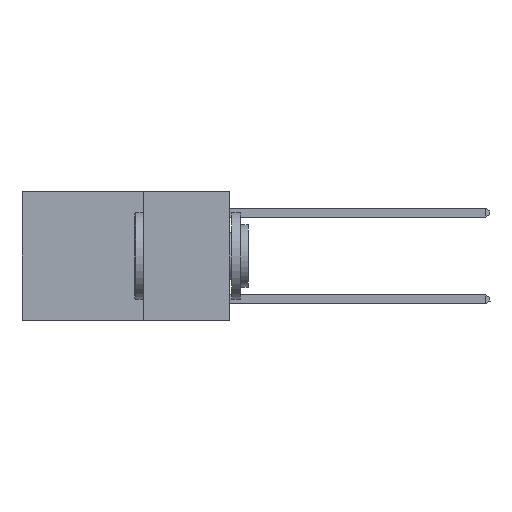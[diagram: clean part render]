
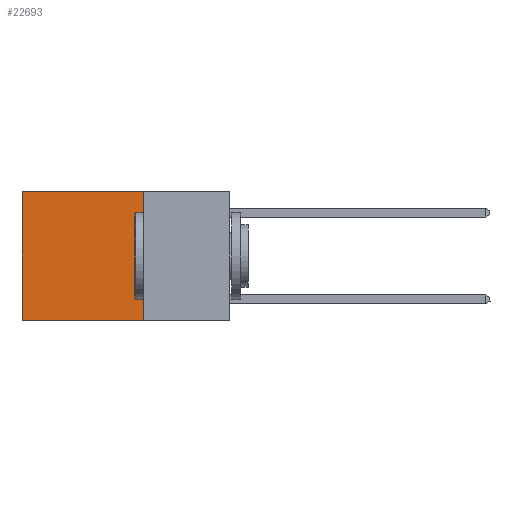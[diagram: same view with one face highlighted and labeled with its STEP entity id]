
A CAD part, left-side view. The second image highlights one B-rep face of the part: STEP entity #22693.
In plain terms, the highlighted planar face has unit normal (-1, 0, 0).
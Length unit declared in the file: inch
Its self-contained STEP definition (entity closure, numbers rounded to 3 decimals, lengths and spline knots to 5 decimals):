
#644 = DIRECTION ( 'NONE',  ( 0., 0., -1. ) ) ;
#819 = VERTEX_POINT ( 'NONE', #11816 ) ;
#1223 = ORIENTED_EDGE ( 'NONE', *, *, #17885, .T. ) ;
#1637 = CARTESIAN_POINT ( 'NONE',  ( 0.2625, 0.25, -0.37 ) ) ;
#1646 = AXIS2_PLACEMENT_3D ( 'NONE', #3803, #3889, #17180 ) ;
#2831 = FACE_OUTER_BOUND ( 'NONE', #8280, .T. ) ;
#3621 = ORIENTED_EDGE ( 'NONE', *, *, #10763, .T. ) ;
#3803 = CARTESIAN_POINT ( 'NONE',  ( 0.2625, 0.25, 0. ) ) ;
#3889 = DIRECTION ( 'NONE',  ( 1., 0., 0. ) ) ;
#4057 = VECTOR ( 'NONE', #19672, 39.37008 ) ;
#4524 = VECTOR ( 'NONE', #24058, 39.37008 ) ;
#4851 = VECTOR ( 'NONE', #5383, 39.37008 ) ;
#5383 = DIRECTION ( 'NONE',  ( 0., 1., 0. ) ) ;
#7064 = EDGE_CURVE ( 'NONE', #819, #14269, #14065, .T. ) ;
#8280 = EDGE_LOOP ( 'NONE', ( #3621, #18998, #20143, #1223 ) ) ;
#8314 = CARTESIAN_POINT ( 'NONE',  ( 0.2625, 0.6, 0. ) ) ;
#10763 = EDGE_CURVE ( 'NONE', #12562, #13441, #23705, .T. ) ;
#11170 = LINE ( 'NONE', #16757, #4851 ) ;
#11816 = CARTESIAN_POINT ( 'NONE',  ( 0.2625, 0.25, 0. ) ) ;
#12133 = CARTESIAN_POINT ( 'NONE',  ( 0.2625, 0.6, 0. ) ) ;
#12462 = CARTESIAN_POINT ( 'NONE',  ( 0.2625, 0.6, -0.37 ) ) ;
#12562 = VERTEX_POINT ( 'NONE', #8314 ) ;
#13441 = VERTEX_POINT ( 'NONE', #12462 ) ;
#13797 = VECTOR ( 'NONE', #644, 39.37008 ) ;
#14065 = LINE ( 'NONE', #22155, #4524 ) ;
#14269 = VERTEX_POINT ( 'NONE', #1637 ) ;
#16757 = CARTESIAN_POINT ( 'NONE',  ( 0.2625, 0.25, 0. ) ) ;
#17180 = DIRECTION ( 'NONE',  ( 0., 0., -1. ) ) ;
#17791 = CARTESIAN_POINT ( 'NONE',  ( 0.2625, 0.25, -0.37 ) ) ;
#17885 = EDGE_CURVE ( 'NONE', #819, #12562, #11170, .T. ) ;
#18998 = ORIENTED_EDGE ( 'NONE', *, *, #22177, .F. ) ;
#19196 = LINE ( 'NONE', #17791, #4057 ) ;
#19672 = DIRECTION ( 'NONE',  ( 0., 1., 0. ) ) ;
#20143 = ORIENTED_EDGE ( 'NONE', *, *, #7064, .F. ) ;
#22155 = CARTESIAN_POINT ( 'NONE',  ( 0.2625, 0.25, 0. ) ) ;
#22177 = EDGE_CURVE ( 'NONE', #14269, #13441, #19196, .T. ) ;
#22693 = ADVANCED_FACE ( 'NONE', ( #2831 ), #22705, .F. ) ;
#22705 = PLANE ( 'NONE',  #1646 ) ;
#23705 = LINE ( 'NONE', #12133, #13797 ) ;
#24058 = DIRECTION ( 'NONE',  ( 0., 0., -1. ) ) ;
